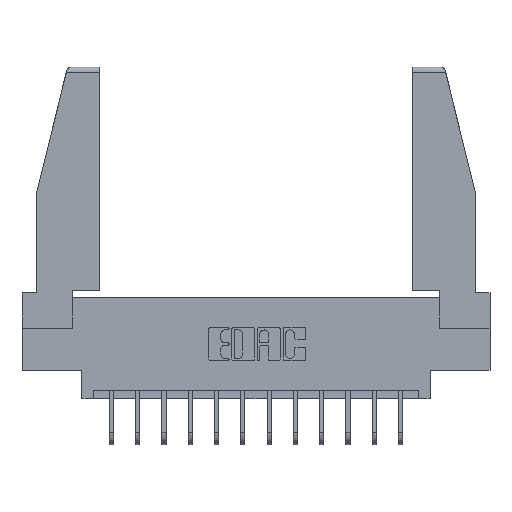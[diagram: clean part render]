
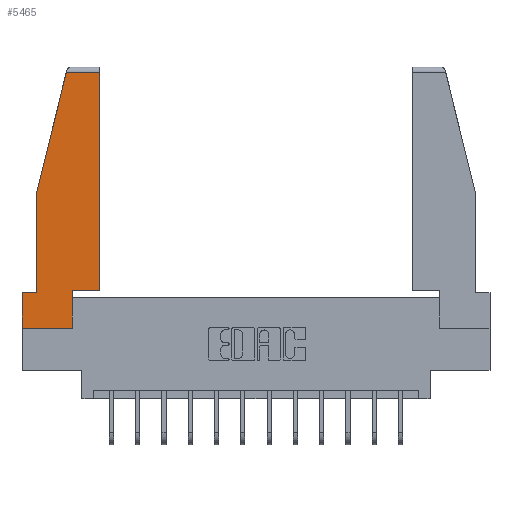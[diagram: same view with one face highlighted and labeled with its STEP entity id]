
A CAD part, top view. The second image highlights one B-rep face of the part: STEP entity #5465.
In plain terms, the highlighted planar face has unit normal (0, 0, 1).
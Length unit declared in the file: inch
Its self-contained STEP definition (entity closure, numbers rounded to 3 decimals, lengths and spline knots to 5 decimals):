
#89 = CARTESIAN_POINT ( 'NONE',  ( 0., 0., 0. ) ) ;
#177 = EDGE_CURVE ( 'NONE', #11490, #11421, #12057, .T. ) ;
#343 = EDGE_CURVE ( 'NONE', #1762, #8163, #1704, .T. ) ;
#543 = ORIENTED_EDGE ( 'NONE', *, *, #12494, .T. ) ;
#718 = ORIENTED_EDGE ( 'NONE', *, *, #11372, .T. ) ;
#723 = CARTESIAN_POINT ( 'NONE',  ( 0.297, 0.223, 0. ) ) ;
#1051 = DIRECTION ( 'NONE',  ( 0., 0., 1. ) ) ;
#1156 = CARTESIAN_POINT ( 'NONE',  ( 0., 0., 0. ) ) ;
#1204 = CARTESIAN_POINT ( 'NONE',  ( 0.297, 0., 0. ) ) ;
#1243 = DIRECTION ( 'NONE',  ( 1., 0., 0. ) ) ;
#1704 = LINE ( 'NONE', #15443, #11231 ) ;
#1762 = VERTEX_POINT ( 'NONE', #7876 ) ;
#1894 = EDGE_LOOP ( 'NONE', ( #5278, #543, #718, #16470, #3141, #6969, #6453, #10364, #15179 ) ) ;
#2038 = CARTESIAN_POINT ( 'NONE',  ( 0., 0.21, 0. ) ) ;
#2120 = CARTESIAN_POINT ( 'NONE',  ( 0.461, 1.52, 0. ) ) ;
#2202 = VECTOR ( 'NONE', #13235, 39.37008 ) ;
#2564 = LINE ( 'NONE', #12744, #13819 ) ;
#3141 = ORIENTED_EDGE ( 'NONE', *, *, #177, .T. ) ;
#3162 = FACE_OUTER_BOUND ( 'NONE', #1894, .T. ) ;
#3164 = VECTOR ( 'NONE', #13873, 39.37008 ) ;
#3172 = EDGE_CURVE ( 'NONE', #6426, #11490, #12971, .T. ) ;
#3533 = DIRECTION ( 'NONE',  ( -1., 0., 0. ) ) ;
#3569 = LINE ( 'NONE', #1156, #12255 ) ;
#4006 = CARTESIAN_POINT ( 'NONE',  ( 0.297, 0., 0. ) ) ;
#4028 = CARTESIAN_POINT ( 'NONE',  ( 0.086, 0.21, 0. ) ) ;
#4079 = LINE ( 'NONE', #1204, #5548 ) ;
#4949 = DIRECTION ( 'NONE',  ( 1., 0., 0. ) ) ;
#5249 = VECTOR ( 'NONE', #3533, 39.37008 ) ;
#5278 = ORIENTED_EDGE ( 'NONE', *, *, #343, .T. ) ;
#5330 = CARTESIAN_POINT ( 'NONE',  ( 0.086, 0.8, 0. ) ) ;
#5465 = ADVANCED_FACE ( 'NONE', ( #3162 ), #17252, .T. ) ;
#5466 = CARTESIAN_POINT ( 'NONE',  ( 0., 0.21, 0. ) ) ;
#5548 = VECTOR ( 'NONE', #16215, 39.37008 ) ;
#5616 = EDGE_CURVE ( 'NONE', #13787, #12067, #3569, .T. ) ;
#6017 = CARTESIAN_POINT ( 'NONE',  ( 0.297, 0.223, 0. ) ) ;
#6090 = LINE ( 'NONE', #6017, #8689 ) ;
#6426 = VERTEX_POINT ( 'NONE', #8642 ) ;
#6453 = ORIENTED_EDGE ( 'NONE', *, *, #5616, .T. ) ;
#6969 = ORIENTED_EDGE ( 'NONE', *, *, #14340, .T. ) ;
#7876 = CARTESIAN_POINT ( 'NONE',  ( 0.461, 0.223, 0. ) ) ;
#8163 = VERTEX_POINT ( 'NONE', #2120 ) ;
#8642 = CARTESIAN_POINT ( 'NONE',  ( 0.086, 0.8, 0. ) ) ;
#8689 = VECTOR ( 'NONE', #4949, 39.37008 ) ;
#8756 = VERTEX_POINT ( 'NONE', #13563 ) ;
#8884 = LINE ( 'NONE', #11647, #5249 ) ;
#9104 = CARTESIAN_POINT ( 'NONE',  ( 0., 0., 0. ) ) ;
#9659 = VECTOR ( 'NONE', #14126, 39.37008 ) ;
#10088 = DIRECTION ( 'NONE',  ( 0., 1., 0. ) ) ;
#10364 = ORIENTED_EDGE ( 'NONE', *, *, #16316, .T. ) ;
#11231 = VECTOR ( 'NONE', #10088, 39.37008 ) ;
#11372 = EDGE_CURVE ( 'NONE', #8756, #6426, #2564, .T. ) ;
#11417 = DIRECTION ( 'NONE',  ( -0.239, -0.971, 0. ) ) ;
#11421 = VERTEX_POINT ( 'NONE', #11862 ) ;
#11490 = VERTEX_POINT ( 'NONE', #4028 ) ;
#11647 = CARTESIAN_POINT ( 'NONE',  ( 0., 1.52, 0. ) ) ;
#11862 = CARTESIAN_POINT ( 'NONE',  ( 0., 0.21, 0. ) ) ;
#11926 = EDGE_CURVE ( 'NONE', #13090, #1762, #6090, .T. ) ;
#12057 = LINE ( 'NONE', #5466, #3164 ) ;
#12067 = VERTEX_POINT ( 'NONE', #4006 ) ;
#12255 = VECTOR ( 'NONE', #12270, 39.37008 ) ;
#12270 = DIRECTION ( 'NONE',  ( 1., 0., 0. ) ) ;
#12494 = EDGE_CURVE ( 'NONE', #8163, #8756, #8884, .T. ) ;
#12744 = CARTESIAN_POINT ( 'NONE',  ( 0.271, 1.55, 0. ) ) ;
#12971 = LINE ( 'NONE', #5330, #2202 ) ;
#13090 = VERTEX_POINT ( 'NONE', #723 ) ;
#13235 = DIRECTION ( 'NONE',  ( 0., -1., 0. ) ) ;
#13246 = LINE ( 'NONE', #2038, #9659 ) ;
#13563 = CARTESIAN_POINT ( 'NONE',  ( 0.2636, 1.52, 0. ) ) ;
#13787 = VERTEX_POINT ( 'NONE', #89 ) ;
#13819 = VECTOR ( 'NONE', #11417, 39.37008 ) ;
#13823 = AXIS2_PLACEMENT_3D ( 'NONE', #9104, #1051, #1243 ) ;
#13873 = DIRECTION ( 'NONE',  ( -1., 0., 0. ) ) ;
#14126 = DIRECTION ( 'NONE',  ( 0., -1., 0. ) ) ;
#14340 = EDGE_CURVE ( 'NONE', #11421, #13787, #13246, .T. ) ;
#15179 = ORIENTED_EDGE ( 'NONE', *, *, #11926, .T. ) ;
#15443 = CARTESIAN_POINT ( 'NONE',  ( 0.461, 0.223, 0. ) ) ;
#16215 = DIRECTION ( 'NONE',  ( 0., 1., 0. ) ) ;
#16316 = EDGE_CURVE ( 'NONE', #12067, #13090, #4079, .T. ) ;
#16470 = ORIENTED_EDGE ( 'NONE', *, *, #3172, .T. ) ;
#17252 = PLANE ( 'NONE',  #13823 ) ;
